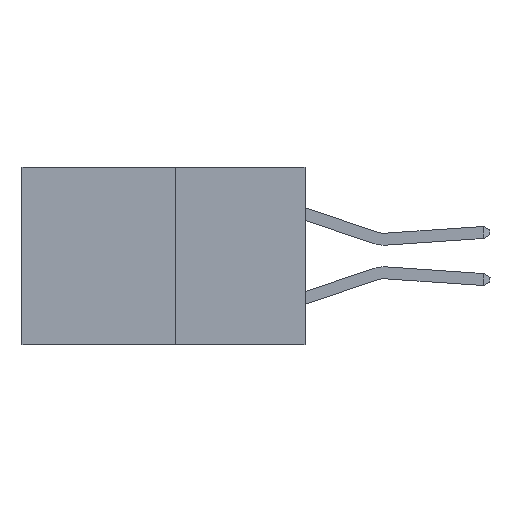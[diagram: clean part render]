
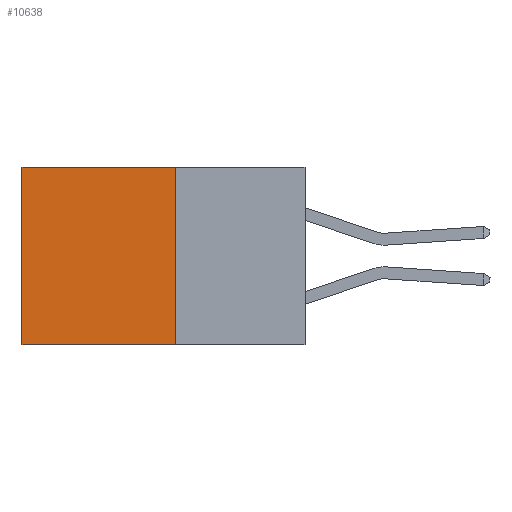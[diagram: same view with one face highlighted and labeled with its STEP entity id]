
A CAD part, left-side view. The second image highlights one B-rep face of the part: STEP entity #10638.
In plain terms, the highlighted planar face has unit normal (-1, 0, 0).
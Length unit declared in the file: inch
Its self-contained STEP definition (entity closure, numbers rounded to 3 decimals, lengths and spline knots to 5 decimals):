
#1912 = CARTESIAN_POINT ( 'NONE',  ( 0.277, 0.59, 0. ) ) ;
#3647 = EDGE_CURVE ( 'NONE', #11009, #27029, #28840, .T. ) ;
#5152 = CARTESIAN_POINT ( 'NONE',  ( 0.277, 0.27, 0. ) ) ;
#5322 = ORIENTED_EDGE ( 'NONE', *, *, #24934, .F. ) ;
#7731 = DIRECTION ( 'NONE',  ( 0., 1., 0. ) ) ;
#8526 = ORIENTED_EDGE ( 'NONE', *, *, #3647, .F. ) ;
#9772 = VECTOR ( 'NONE', #31974, 39.37008 ) ;
#10638 = ADVANCED_FACE ( 'NONE', ( #20327 ), #30106, .F. ) ;
#10772 = AXIS2_PLACEMENT_3D ( 'NONE', #29938, #29868, #29860 ) ;
#11009 = VERTEX_POINT ( 'NONE', #19859 ) ;
#11999 = DIRECTION ( 'NONE',  ( 0., 0., -1. ) ) ;
#12078 = VECTOR ( 'NONE', #11999, 39.37008 ) ;
#13000 = EDGE_LOOP ( 'NONE', ( #29669, #5322, #8526, #29035 ) ) ;
#14369 = LINE ( 'NONE', #5152, #26868 ) ;
#15216 = VERTEX_POINT ( 'NONE', #25061 ) ;
#16377 = VERTEX_POINT ( 'NONE', #1912 ) ;
#18408 = LINE ( 'NONE', #29420, #12078 ) ;
#18527 = CARTESIAN_POINT ( 'NONE',  ( 0.277, 0.27, -0.37 ) ) ;
#19129 = EDGE_CURVE ( 'NONE', #16377, #15216, #18408, .T. ) ;
#19859 = CARTESIAN_POINT ( 'NONE',  ( 0.277, 0.27, 0. ) ) ;
#20327 = FACE_OUTER_BOUND ( 'NONE', #13000, .T. ) ;
#21269 = LINE ( 'NONE', #18527, #27047 ) ;
#24934 = EDGE_CURVE ( 'NONE', #27029, #15216, #21269, .T. ) ;
#25061 = CARTESIAN_POINT ( 'NONE',  ( 0.277, 0.59, -0.37 ) ) ;
#26015 = DIRECTION ( 'NONE',  ( 0., 1., 0. ) ) ;
#26868 = VECTOR ( 'NONE', #7731, 39.37008 ) ;
#27029 = VERTEX_POINT ( 'NONE', #31388 ) ;
#27047 = VECTOR ( 'NONE', #26015, 39.37008 ) ;
#28289 = EDGE_CURVE ( 'NONE', #11009, #16377, #14369, .T. ) ;
#28840 = LINE ( 'NONE', #30937, #9772 ) ;
#29035 = ORIENTED_EDGE ( 'NONE', *, *, #28289, .T. ) ;
#29420 = CARTESIAN_POINT ( 'NONE',  ( 0.277, 0.59, -0.37 ) ) ;
#29669 = ORIENTED_EDGE ( 'NONE', *, *, #19129, .T. ) ;
#29860 = DIRECTION ( 'NONE',  ( 0., 0., -1. ) ) ;
#29868 = DIRECTION ( 'NONE',  ( 1., 0., 0. ) ) ;
#29938 = CARTESIAN_POINT ( 'NONE',  ( 0.277, 0.27, -0.37 ) ) ;
#30106 = PLANE ( 'NONE',  #10772 ) ;
#30937 = CARTESIAN_POINT ( 'NONE',  ( 0.277, 0.27, -0.37 ) ) ;
#31388 = CARTESIAN_POINT ( 'NONE',  ( 0.277, 0.27, -0.37 ) ) ;
#31974 = DIRECTION ( 'NONE',  ( 0., 0., -1. ) ) ;
